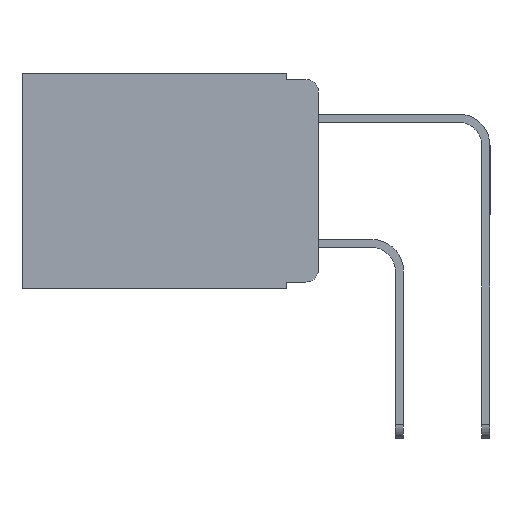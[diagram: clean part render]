
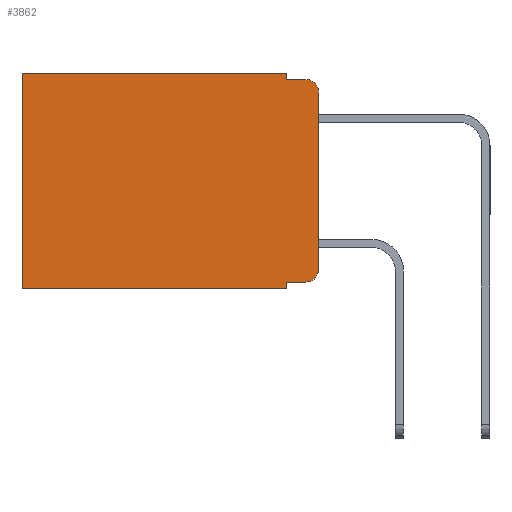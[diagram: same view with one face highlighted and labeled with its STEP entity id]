
A CAD part, left-side view. The second image highlights one B-rep face of the part: STEP entity #3862.
In plain terms, the highlighted planar face has unit normal (-1, 0, 0).
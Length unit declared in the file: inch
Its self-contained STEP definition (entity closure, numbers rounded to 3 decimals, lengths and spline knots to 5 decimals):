
#138 = CARTESIAN_POINT ( 'NONE',  ( 0.298, 0.473, 0. ) ) ;
#413 = CARTESIAN_POINT ( 'NONE',  ( 0.298, 0., -0.343 ) ) ;
#714 = EDGE_CURVE ( 'NONE', #11237, #21530, #10503, .T. ) ;
#771 = CARTESIAN_POINT ( 'NONE',  ( 0.298, 0.051, -0.333 ) ) ;
#1806 = LINE ( 'NONE', #14964, #6080 ) ;
#1897 = VERTEX_POINT ( 'NONE', #771 ) ;
#2110 = DIRECTION ( 'NONE',  ( 0., 0., -1. ) ) ;
#2637 = ORIENTED_EDGE ( 'NONE', *, *, #14778, .F. ) ;
#2717 = ORIENTED_EDGE ( 'NONE', *, *, #7566, .F. ) ;
#2783 = LINE ( 'NONE', #22120, #7002 ) ;
#2886 = VECTOR ( 'NONE', #8477, 39.37008 ) ;
#2967 = VECTOR ( 'NONE', #9150, 39.37008 ) ;
#3299 = VECTOR ( 'NONE', #2110, 39.37008 ) ;
#3407 = VECTOR ( 'NONE', #20961, 39.37008 ) ;
#3421 = ORIENTED_EDGE ( 'NONE', *, *, #714, .T. ) ;
#3862 = ADVANCED_FACE ( 'NONE', ( #4810 ), #19618, .F. ) ;
#4000 = CARTESIAN_POINT ( 'NONE',  ( 0.298, 0.051, -0.343 ) ) ;
#4199 = DIRECTION ( 'NONE',  ( -1., 0., 0. ) ) ;
#4360 = DIRECTION ( 'NONE',  ( 0., 1., 0. ) ) ;
#4593 = EDGE_CURVE ( 'NONE', #11709, #8629, #10633, .T. ) ;
#4810 = FACE_OUTER_BOUND ( 'NONE', #18018, .T. ) ;
#4844 = CARTESIAN_POINT ( 'NONE',  ( 0.298, 0., 0. ) ) ;
#5183 = ORIENTED_EDGE ( 'NONE', *, *, #8909, .F. ) ;
#5557 = CARTESIAN_POINT ( 'NONE',  ( 0.298, 0.051, 0. ) ) ;
#6080 = VECTOR ( 'NONE', #6181, 39.37008 ) ;
#6181 = DIRECTION ( 'NONE',  ( 0., 0., -1. ) ) ;
#7002 = VECTOR ( 'NONE', #13669, 39.37008 ) ;
#7268 = VERTEX_POINT ( 'NONE', #15772 ) ;
#7566 = EDGE_CURVE ( 'NONE', #11201, #15797, #21718, .T. ) ;
#8012 = VECTOR ( 'NONE', #4360, 39.37008 ) ;
#8477 = DIRECTION ( 'NONE',  ( 0., -1., 0. ) ) ;
#8629 = VERTEX_POINT ( 'NONE', #14197 ) ;
#8869 = CARTESIAN_POINT ( 'NONE',  ( 0.298, 0.02, -0.313 ) ) ;
#8908 = VERTEX_POINT ( 'NONE', #18210 ) ;
#8909 = EDGE_CURVE ( 'NONE', #1897, #11201, #1806, .T. ) ;
#9006 = VECTOR ( 'NONE', #15409, 39.37008 ) ;
#9150 = DIRECTION ( 'NONE',  ( 0., 0., -1. ) ) ;
#9229 = VERTEX_POINT ( 'NONE', #19199 ) ;
#9888 = DIRECTION ( 'NONE',  ( -1., 0., 0. ) ) ;
#10288 = CIRCLE ( 'NONE', #10880, 0.02 ) ;
#10503 = CIRCLE ( 'NONE', #19665, 0.02 ) ;
#10633 = LINE ( 'NONE', #4844, #9006 ) ;
#10880 = AXIS2_PLACEMENT_3D ( 'NONE', #20166, #9888, #21852 ) ;
#11201 = VERTEX_POINT ( 'NONE', #4000 ) ;
#11202 = CARTESIAN_POINT ( 'NONE',  ( 0.298, 0.02, -0.333 ) ) ;
#11237 = VERTEX_POINT ( 'NONE', #11202 ) ;
#11603 = CARTESIAN_POINT ( 'NONE',  ( 0.298, 0.473, -0.343 ) ) ;
#11709 = VERTEX_POINT ( 'NONE', #14543 ) ;
#11900 = ORIENTED_EDGE ( 'NONE', *, *, #22661, .F. ) ;
#12730 = LINE ( 'NONE', #138, #3299 ) ;
#13578 = EDGE_CURVE ( 'NONE', #8629, #15797, #12730, .T. ) ;
#13669 = DIRECTION ( 'NONE',  ( 0., -1., 0. ) ) ;
#13701 = DIRECTION ( 'NONE',  ( 0., 0., -1. ) ) ;
#14168 = CARTESIAN_POINT ( 'NONE',  ( 0.298, 0., 0. ) ) ;
#14197 = CARTESIAN_POINT ( 'NONE',  ( 0.298, 0.473, 0. ) ) ;
#14499 = ORIENTED_EDGE ( 'NONE', *, *, #21856, .T. ) ;
#14543 = CARTESIAN_POINT ( 'NONE',  ( 0.298, 0.051, 0. ) ) ;
#14609 = CARTESIAN_POINT ( 'NONE',  ( 0.298, 0., -0.313 ) ) ;
#14778 = EDGE_CURVE ( 'NONE', #11709, #8908, #17010, .T. ) ;
#14964 = CARTESIAN_POINT ( 'NONE',  ( 0.298, 0.051, 0. ) ) ;
#15409 = DIRECTION ( 'NONE',  ( 0., 1., 0. ) ) ;
#15772 = CARTESIAN_POINT ( 'NONE',  ( 0.298, 0.02, -0.01 ) ) ;
#15797 = VERTEX_POINT ( 'NONE', #11603 ) ;
#15915 = EDGE_CURVE ( 'NONE', #8908, #7268, #2783, .T. ) ;
#16252 = ORIENTED_EDGE ( 'NONE', *, *, #17053, .T. ) ;
#17010 = LINE ( 'NONE', #5557, #2967 ) ;
#17053 = EDGE_CURVE ( 'NONE', #9229, #7268, #10288, .T. ) ;
#17206 = CARTESIAN_POINT ( 'NONE',  ( 0.298, 0.051, -0.333 ) ) ;
#17423 = LINE ( 'NONE', #14168, #3407 ) ;
#17468 = LINE ( 'NONE', #17206, #2886 ) ;
#17786 = CARTESIAN_POINT ( 'NONE',  ( 0.298, 0., 0. ) ) ;
#18018 = EDGE_LOOP ( 'NONE', ( #11900, #16252, #21080, #2637, #20889, #22801, #2717, #5183, #14499, #3421 ) ) ;
#18210 = CARTESIAN_POINT ( 'NONE',  ( 0.298, 0.051, -0.01 ) ) ;
#19199 = CARTESIAN_POINT ( 'NONE',  ( 0.298, 0., -0.03 ) ) ;
#19563 = DIRECTION ( 'NONE',  ( 1., 0., 0. ) ) ;
#19618 = PLANE ( 'NONE',  #22233 ) ;
#19665 = AXIS2_PLACEMENT_3D ( 'NONE', #8869, #4199, #13701 ) ;
#20166 = CARTESIAN_POINT ( 'NONE',  ( 0.298, 0.02, -0.03 ) ) ;
#20889 = ORIENTED_EDGE ( 'NONE', *, *, #4593, .T. ) ;
#20961 = DIRECTION ( 'NONE',  ( 0., 0., -1. ) ) ;
#21080 = ORIENTED_EDGE ( 'NONE', *, *, #15915, .F. ) ;
#21530 = VERTEX_POINT ( 'NONE', #14609 ) ;
#21718 = LINE ( 'NONE', #413, #8012 ) ;
#21852 = DIRECTION ( 'NONE',  ( 0., 0., -1. ) ) ;
#21856 = EDGE_CURVE ( 'NONE', #1897, #11237, #17468, .T. ) ;
#22120 = CARTESIAN_POINT ( 'NONE',  ( 0.298, 0.051, -0.01 ) ) ;
#22233 = AXIS2_PLACEMENT_3D ( 'NONE', #17786, #19563, #22748 ) ;
#22661 = EDGE_CURVE ( 'NONE', #9229, #21530, #17423, .T. ) ;
#22748 = DIRECTION ( 'NONE',  ( 0., 0., -1. ) ) ;
#22801 = ORIENTED_EDGE ( 'NONE', *, *, #13578, .T. ) ;
